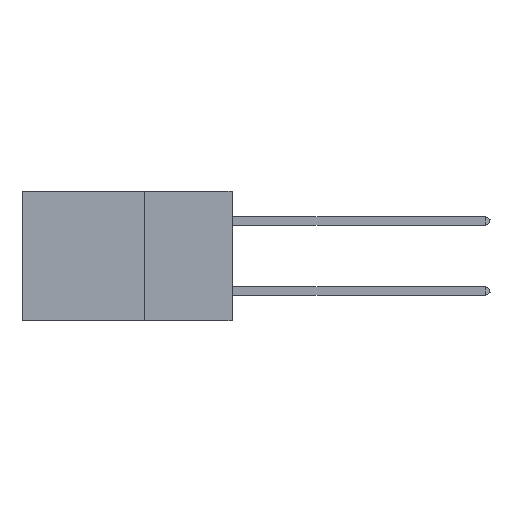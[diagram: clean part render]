
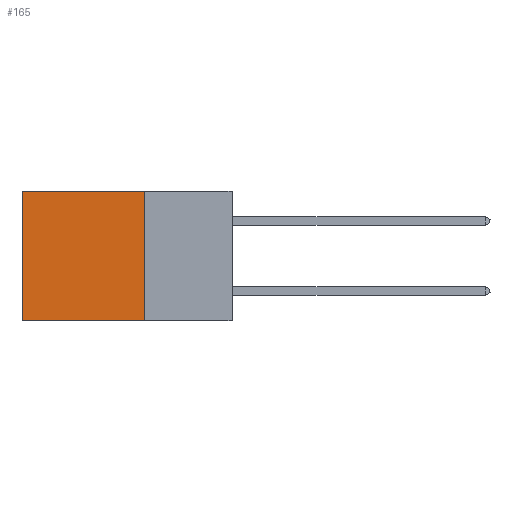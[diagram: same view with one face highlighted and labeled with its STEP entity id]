
A CAD part, left-side view. The second image highlights one B-rep face of the part: STEP entity #165.
In plain terms, the highlighted planar face has unit normal (-1, 0, 0).
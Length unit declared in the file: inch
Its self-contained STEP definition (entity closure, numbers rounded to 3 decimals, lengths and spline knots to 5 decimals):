
#119 = CARTESIAN_POINT ( 'NONE',  ( 0.2875, 0.25, 0. ) ) ;
#165 = ADVANCED_FACE ( 'NONE', ( #8215 ), #21221, .F. ) ;
#796 = CARTESIAN_POINT ( 'NONE',  ( 0.2875, 0.25, 0. ) ) ;
#1224 = EDGE_CURVE ( 'NONE', #22248, #46346, #30005, .T. ) ;
#1354 = DIRECTION ( 'NONE',  ( 0., 0., -1. ) ) ;
#2644 = VERTEX_POINT ( 'NONE', #39119 ) ;
#3280 = EDGE_CURVE ( 'NONE', #35888, #2644, #33661, .T. ) ;
#6533 = VECTOR ( 'NONE', #31546, 39.37008 ) ;
#8215 = FACE_OUTER_BOUND ( 'NONE', #13066, .T. ) ;
#10185 = ORIENTED_EDGE ( 'NONE', *, *, #37203, .F. ) ;
#11586 = AXIS2_PLACEMENT_3D ( 'NONE', #35831, #46864, #24903 ) ;
#13066 = EDGE_LOOP ( 'NONE', ( #17130, #27286, #10185, #25307 ) ) ;
#14161 = DIRECTION ( 'NONE',  ( 0., 0., -1. ) ) ;
#16024 = LINE ( 'NONE', #23586, #35512 ) ;
#16947 = CARTESIAN_POINT ( 'NONE',  ( 0.2875, 0.25, -0.37 ) ) ;
#17130 = ORIENTED_EDGE ( 'NONE', *, *, #40266, .T. ) ;
#19081 = VECTOR ( 'NONE', #26764, 39.37008 ) ;
#20806 = CARTESIAN_POINT ( 'NONE',  ( 0.2875, 0.25, -0.37 ) ) ;
#21221 = PLANE ( 'NONE',  #11586 ) ;
#22248 = VERTEX_POINT ( 'NONE', #119 ) ;
#23586 = CARTESIAN_POINT ( 'NONE',  ( 0.2875, 0.6, 0. ) ) ;
#24903 = DIRECTION ( 'NONE',  ( 0., 0., -1. ) ) ;
#25307 = ORIENTED_EDGE ( 'NONE', *, *, #1224, .T. ) ;
#26672 = CARTESIAN_POINT ( 'NONE',  ( 0.2875, 0.6, 0. ) ) ;
#26764 = DIRECTION ( 'NONE',  ( 0., 1., 0. ) ) ;
#27286 = ORIENTED_EDGE ( 'NONE', *, *, #3280, .F. ) ;
#30005 = LINE ( 'NONE', #796, #19081 ) ;
#31546 = DIRECTION ( 'NONE',  ( 0., 1., 0. ) ) ;
#33661 = LINE ( 'NONE', #16947, #6533 ) ;
#35512 = VECTOR ( 'NONE', #1354, 39.37008 ) ;
#35831 = CARTESIAN_POINT ( 'NONE',  ( 0.2875, 0.25, 0. ) ) ;
#35888 = VERTEX_POINT ( 'NONE', #20806 ) ;
#37203 = EDGE_CURVE ( 'NONE', #22248, #35888, #42588, .T. ) ;
#39119 = CARTESIAN_POINT ( 'NONE',  ( 0.2875, 0.6, -0.37 ) ) ;
#40266 = EDGE_CURVE ( 'NONE', #46346, #2644, #16024, .T. ) ;
#40280 = VECTOR ( 'NONE', #14161, 39.37008 ) ;
#42588 = LINE ( 'NONE', #46979, #40280 ) ;
#46346 = VERTEX_POINT ( 'NONE', #26672 ) ;
#46864 = DIRECTION ( 'NONE',  ( 1., 0., 0. ) ) ;
#46979 = CARTESIAN_POINT ( 'NONE',  ( 0.2875, 0.25, 0. ) ) ;
